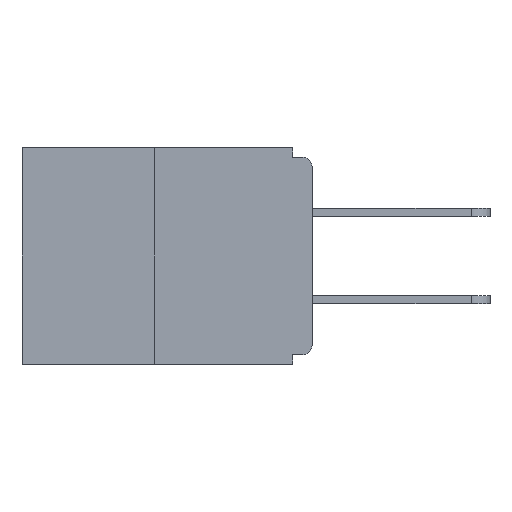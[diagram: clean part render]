
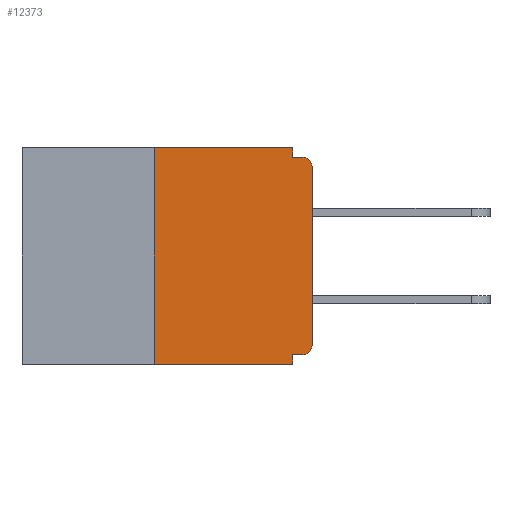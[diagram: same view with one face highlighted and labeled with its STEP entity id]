
A CAD part, left-side view. The second image highlights one B-rep face of the part: STEP entity #12373.
In plain terms, the highlighted planar face has unit normal (-1, 0, 0).
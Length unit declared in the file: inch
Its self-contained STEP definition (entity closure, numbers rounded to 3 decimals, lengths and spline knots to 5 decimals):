
#395 = VECTOR ( 'NONE', #15963, 39.37008 ) ;
#422 = DIRECTION ( 'NONE',  ( 0., 0., 1. ) ) ;
#514 = EDGE_LOOP ( 'NONE', ( #7778, #9089, #10684, #13365, #3101, #2390, #9456, #14915, #11963, #2451 ) ) ;
#662 = CARTESIAN_POINT ( 'NONE',  ( 0., 0.015, -0.015 ) ) ;
#1963 = CARTESIAN_POINT ( 'NONE',  ( 0., 0.031, -0.343 ) ) ;
#2011 = VERTEX_POINT ( 'NONE', #9145 ) ;
#2303 = CARTESIAN_POINT ( 'NONE',  ( 0., 0.031, -0.343 ) ) ;
#2390 = ORIENTED_EDGE ( 'NONE', *, *, #5406, .T. ) ;
#2408 = DIRECTION ( 'NONE',  ( 0., -1., 0. ) ) ;
#2441 = CARTESIAN_POINT ( 'NONE',  ( 0., 0., -0.328 ) ) ;
#2451 = ORIENTED_EDGE ( 'NONE', *, *, #5545, .F. ) ;
#3101 = ORIENTED_EDGE ( 'NONE', *, *, #14983, .F. ) ;
#3498 = DIRECTION ( 'NONE',  ( 0., 0., -1. ) ) ;
#3553 = CARTESIAN_POINT ( 'NONE',  ( 0., 0.031, 0. ) ) ;
#3813 = DIRECTION ( 'NONE',  ( 0., 0., -1. ) ) ;
#4040 = CIRCLE ( 'NONE', #16617, 0.015 ) ;
#4273 = VERTEX_POINT ( 'NONE', #662 ) ;
#4569 = VERTEX_POINT ( 'NONE', #10979 ) ;
#5394 = CARTESIAN_POINT ( 'NONE',  ( 0., 0., -0.03 ) ) ;
#5406 = EDGE_CURVE ( 'NONE', #14177, #6668, #14106, .T. ) ;
#5545 = EDGE_CURVE ( 'NONE', #6407, #2011, #14538, .T. ) ;
#5581 = DIRECTION ( 'NONE',  ( 0., 0., -1. ) ) ;
#5605 = EDGE_CURVE ( 'NONE', #6334, #9056, #10723, .T. ) ;
#5738 = CARTESIAN_POINT ( 'NONE',  ( 0., 0., 0. ) ) ;
#5784 = VECTOR ( 'NONE', #422, 39.37008 ) ;
#6017 = LINE ( 'NONE', #7469, #14694 ) ;
#6307 = EDGE_CURVE ( 'NONE', #4569, #6407, #12713, .T. ) ;
#6334 = VERTEX_POINT ( 'NONE', #17574 ) ;
#6407 = VERTEX_POINT ( 'NONE', #9376 ) ;
#6668 = VERTEX_POINT ( 'NONE', #8591 ) ;
#6836 = FACE_OUTER_BOUND ( 'NONE', #514, .T. ) ;
#7259 = LINE ( 'NONE', #14212, #14059 ) ;
#7366 = DIRECTION ( 'NONE',  ( -1., 0., 0. ) ) ;
#7460 = CARTESIAN_POINT ( 'NONE',  ( 0., 0.46, 0. ) ) ;
#7469 = CARTESIAN_POINT ( 'NONE',  ( 0., 0.46, -0.343 ) ) ;
#7778 = ORIENTED_EDGE ( 'NONE', *, *, #6307, .F. ) ;
#8591 = CARTESIAN_POINT ( 'NONE',  ( 0., 0., -0.313 ) ) ;
#8820 = DIRECTION ( 'NONE',  ( 0., 0., 1. ) ) ;
#9056 = VERTEX_POINT ( 'NONE', #1963 ) ;
#9089 = ORIENTED_EDGE ( 'NONE', *, *, #10255, .F. ) ;
#9145 = CARTESIAN_POINT ( 'NONE',  ( 0., 0.031, -0.015 ) ) ;
#9341 = LINE ( 'NONE', #11750, #395 ) ;
#9376 = CARTESIAN_POINT ( 'NONE',  ( 0., 0.031, 0. ) ) ;
#9456 = ORIENTED_EDGE ( 'NONE', *, *, #10975, .T. ) ;
#9657 = EDGE_CURVE ( 'NONE', #9896, #9056, #6017, .T. ) ;
#9896 = VERTEX_POINT ( 'NONE', #16233 ) ;
#10255 = EDGE_CURVE ( 'NONE', #9896, #4569, #7259, .T. ) ;
#10545 = LINE ( 'NONE', #2441, #17345 ) ;
#10684 = ORIENTED_EDGE ( 'NONE', *, *, #9657, .T. ) ;
#10723 = LINE ( 'NONE', #2303, #16232 ) ;
#10884 = VERTEX_POINT ( 'NONE', #5394 ) ;
#10975 = EDGE_CURVE ( 'NONE', #6668, #10884, #11500, .T. ) ;
#10979 = CARTESIAN_POINT ( 'NONE',  ( 0., 0.25, 0. ) ) ;
#11199 = CARTESIAN_POINT ( 'NONE',  ( 0., 0.015, -0.03 ) ) ;
#11500 = LINE ( 'NONE', #5738, #5784 ) ;
#11524 = AXIS2_PLACEMENT_3D ( 'NONE', #15419, #7366, #12951 ) ;
#11672 = DIRECTION ( 'NONE',  ( 0., -1., 0. ) ) ;
#11750 = CARTESIAN_POINT ( 'NONE',  ( 0., 0., -0.015 ) ) ;
#11802 = CARTESIAN_POINT ( 'NONE',  ( 0., 0.015, -0.328 ) ) ;
#11963 = ORIENTED_EDGE ( 'NONE', *, *, #13110, .F. ) ;
#12179 = DIRECTION ( 'NONE',  ( 0., 1., 0. ) ) ;
#12373 = ADVANCED_FACE ( 'NONE', ( #6836 ), #14158, .F. ) ;
#12564 = EDGE_CURVE ( 'NONE', #10884, #4273, #4040, .T. ) ;
#12713 = LINE ( 'NONE', #14875, #17396 ) ;
#12951 = DIRECTION ( 'NONE',  ( 0., 0., -1. ) ) ;
#13110 = EDGE_CURVE ( 'NONE', #2011, #4273, #9341, .T. ) ;
#13365 = ORIENTED_EDGE ( 'NONE', *, *, #5605, .F. ) ;
#13679 = VECTOR ( 'NONE', #14544, 39.37008 ) ;
#14059 = VECTOR ( 'NONE', #8820, 39.37008 ) ;
#14106 = CIRCLE ( 'NONE', #11524, 0.015 ) ;
#14158 = PLANE ( 'NONE',  #14798 ) ;
#14177 = VERTEX_POINT ( 'NONE', #11802 ) ;
#14212 = CARTESIAN_POINT ( 'NONE',  ( 0., 0.25, 0. ) ) ;
#14538 = LINE ( 'NONE', #3553, #13679 ) ;
#14544 = DIRECTION ( 'NONE',  ( 0., 0., -1. ) ) ;
#14694 = VECTOR ( 'NONE', #11672, 39.37008 ) ;
#14798 = AXIS2_PLACEMENT_3D ( 'NONE', #7460, #17309, #3813 ) ;
#14875 = CARTESIAN_POINT ( 'NONE',  ( 0., 0.46, 0. ) ) ;
#14915 = ORIENTED_EDGE ( 'NONE', *, *, #12564, .T. ) ;
#14983 = EDGE_CURVE ( 'NONE', #14177, #6334, #10545, .T. ) ;
#15285 = DIRECTION ( 'NONE',  ( -1., 0., 0. ) ) ;
#15419 = CARTESIAN_POINT ( 'NONE',  ( 0., 0.015, -0.313 ) ) ;
#15963 = DIRECTION ( 'NONE',  ( 0., -1., 0. ) ) ;
#16232 = VECTOR ( 'NONE', #3498, 39.37008 ) ;
#16233 = CARTESIAN_POINT ( 'NONE',  ( 0., 0.25, -0.343 ) ) ;
#16617 = AXIS2_PLACEMENT_3D ( 'NONE', #11199, #15285, #5581 ) ;
#17309 = DIRECTION ( 'NONE',  ( 1., 0., 0. ) ) ;
#17345 = VECTOR ( 'NONE', #12179, 39.37008 ) ;
#17396 = VECTOR ( 'NONE', #2408, 39.37008 ) ;
#17574 = CARTESIAN_POINT ( 'NONE',  ( 0., 0.031, -0.328 ) ) ;
